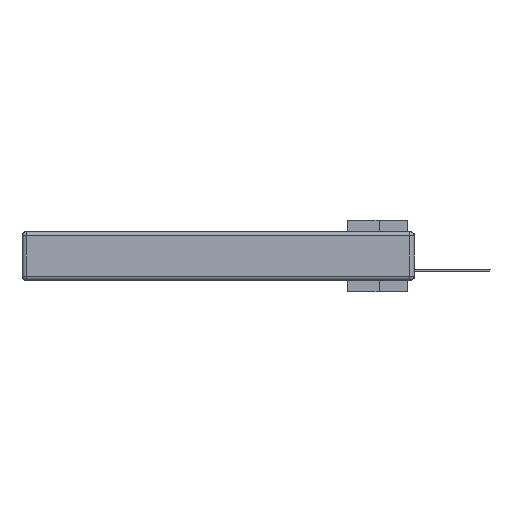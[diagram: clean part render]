
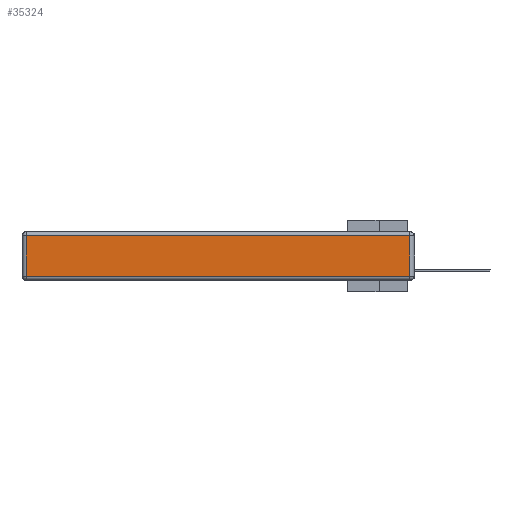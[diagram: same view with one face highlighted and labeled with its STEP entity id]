
A CAD part, left-side view. The second image highlights one B-rep face of the part: STEP entity #35324.
In plain terms, the highlighted planar face has unit normal (-1, 0, 0).
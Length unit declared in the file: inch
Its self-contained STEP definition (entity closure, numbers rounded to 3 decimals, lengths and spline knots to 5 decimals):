
#924 = LINE ( 'NONE', #12926, #12868 ) ;
#3648 = EDGE_CURVE ( 'NONE', #20778, #29170, #14689, .T. ) ;
#4334 = CARTESIAN_POINT ( 'NONE',  ( 0., 2.72, -0.343 ) ) ;
#4413 = CARTESIAN_POINT ( 'NONE',  ( 0., 0.03, -0.343 ) ) ;
#6339 = VECTOR ( 'NONE', #35359, 39.37008 ) ;
#6650 = DIRECTION ( 'NONE',  ( 0., 0., -1. ) ) ;
#7232 = DIRECTION ( 'NONE',  ( 0., 1., 0. ) ) ;
#8062 = FACE_OUTER_BOUND ( 'NONE', #20261, .T. ) ;
#9925 = CARTESIAN_POINT ( 'NONE',  ( 0., 2.75, -0.03 ) ) ;
#10240 = DIRECTION ( 'NONE',  ( -1., 0., 0. ) ) ;
#10520 = EDGE_CURVE ( 'NONE', #29170, #23327, #14728, .T. ) ;
#10579 = EDGE_CURVE ( 'NONE', #23327, #24406, #924, .T. ) ;
#12713 = CARTESIAN_POINT ( 'NONE',  ( 0., 2.72, -0.313 ) ) ;
#12868 = VECTOR ( 'NONE', #22887, 39.37008 ) ;
#12926 = CARTESIAN_POINT ( 'NONE',  ( 0., 0., -0.313 ) ) ;
#14689 = LINE ( 'NONE', #9925, #28771 ) ;
#14728 = LINE ( 'NONE', #4334, #32867 ) ;
#18478 = PLANE ( 'NONE',  #29034 ) ;
#18854 = CARTESIAN_POINT ( 'NONE',  ( 0., 0.03, -0.03 ) ) ;
#20261 = EDGE_LOOP ( 'NONE', ( #36371, #27845, #30082, #27011 ) ) ;
#20778 = VERTEX_POINT ( 'NONE', #18854 ) ;
#22887 = DIRECTION ( 'NONE',  ( 0., -1., 0. ) ) ;
#23327 = VERTEX_POINT ( 'NONE', #12713 ) ;
#24406 = VERTEX_POINT ( 'NONE', #31622 ) ;
#24550 = DIRECTION ( 'NONE',  ( 0., 0., 1. ) ) ;
#26969 = CARTESIAN_POINT ( 'NONE',  ( 0., 0., -0.343 ) ) ;
#27011 = ORIENTED_EDGE ( 'NONE', *, *, #10520, .T. ) ;
#27845 = ORIENTED_EDGE ( 'NONE', *, *, #33155, .T. ) ;
#28771 = VECTOR ( 'NONE', #7232, 39.37008 ) ;
#29034 = AXIS2_PLACEMENT_3D ( 'NONE', #26969, #10240, #24550 ) ;
#29170 = VERTEX_POINT ( 'NONE', #30899 ) ;
#30082 = ORIENTED_EDGE ( 'NONE', *, *, #3648, .T. ) ;
#30899 = CARTESIAN_POINT ( 'NONE',  ( 0., 2.72, -0.03 ) ) ;
#31622 = CARTESIAN_POINT ( 'NONE',  ( 0., 0.03, -0.313 ) ) ;
#32867 = VECTOR ( 'NONE', #6650, 39.37008 ) ;
#33155 = EDGE_CURVE ( 'NONE', #24406, #20778, #36383, .T. ) ;
#35324 = ADVANCED_FACE ( 'NONE', ( #8062 ), #18478, .T. ) ;
#35359 = DIRECTION ( 'NONE',  ( 0., 0., 1. ) ) ;
#36371 = ORIENTED_EDGE ( 'NONE', *, *, #10579, .T. ) ;
#36383 = LINE ( 'NONE', #4413, #6339 ) ;
